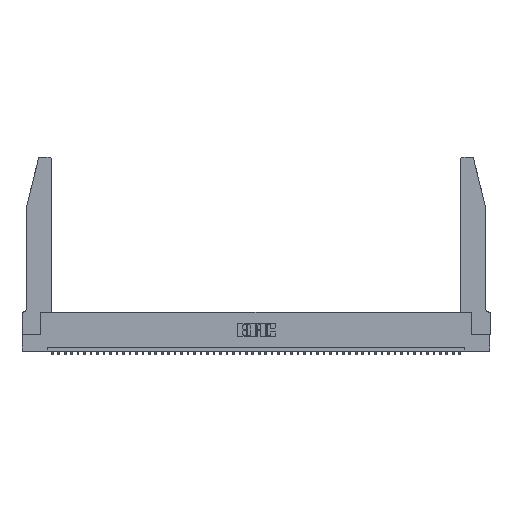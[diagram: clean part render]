
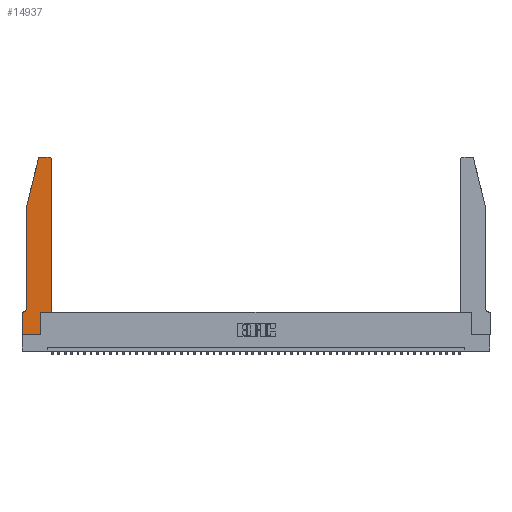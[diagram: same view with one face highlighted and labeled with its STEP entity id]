
A CAD part, top view. The second image highlights one B-rep face of the part: STEP entity #14937.
In plain terms, the highlighted planar face has unit normal (0, 0, 1).
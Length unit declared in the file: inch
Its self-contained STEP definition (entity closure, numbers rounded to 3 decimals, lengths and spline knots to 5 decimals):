
#186 = CARTESIAN_POINT ( 'NONE',  ( 0.0755, 0.35, 0.37 ) ) ;
#230 = AXIS2_PLACEMENT_3D ( 'NONE', #18281, #14562, #41820 ) ;
#433 = DIRECTION ( 'NONE',  ( -0.239, -0.971, 0. ) ) ;
#727 = EDGE_CURVE ( 'NONE', #13771, #45544, #39080, .T. ) ;
#1251 = FACE_OUTER_BOUND ( 'NONE', #7457, .T. ) ;
#2124 = CARTESIAN_POINT ( 'NONE',  ( 0., 0.35, 0.37 ) ) ;
#2493 = EDGE_CURVE ( 'NONE', #27347, #13121, #4326, .T. ) ;
#2676 = VECTOR ( 'NONE', #43701, 39.37008 ) ;
#3773 = CARTESIAN_POINT ( 'NONE',  ( 0.0055, 0.35, 0.37 ) ) ;
#3998 = EDGE_CURVE ( 'NONE', #44544, #13251, #23470, .T. ) ;
#4326 = LINE ( 'NONE', #32568, #39318 ) ;
#4371 = EDGE_CURVE ( 'NONE', #15235, #44544, #29997, .T. ) ;
#4794 = DIRECTION ( 'NONE',  ( 1., 0., 0. ) ) ;
#4804 = ORIENTED_EDGE ( 'NONE', *, *, #6406, .T. ) ;
#5043 = CARTESIAN_POINT ( 'NONE',  ( 0.0755, 2., 0.37 ) ) ;
#6080 = EDGE_CURVE ( 'NONE', #13251, #15840, #48644, .T. ) ;
#6301 = ORIENTED_EDGE ( 'NONE', *, *, #37651, .T. ) ;
#6406 = EDGE_CURVE ( 'NONE', #28997, #15235, #20868, .T. ) ;
#7157 = VECTOR ( 'NONE', #39104, 39.37008 ) ;
#7457 = EDGE_LOOP ( 'NONE', ( #36026, #28416, #6301, #4804, #25164, #46960, #48026, #23947, #49826, #29886, #9608, #45561 ) ) ;
#7654 = CARTESIAN_POINT ( 'NONE',  ( 0., 0., 0.37 ) ) ;
#8870 = CARTESIAN_POINT ( 'NONE',  ( 0.0055, 0.42, 0.37 ) ) ;
#9608 = ORIENTED_EDGE ( 'NONE', *, *, #43253, .T. ) ;
#10741 = EDGE_CURVE ( 'NONE', #34025, #13771, #33424, .T. ) ;
#11911 = CARTESIAN_POINT ( 'NONE',  ( 0., 0., 0.37 ) ) ;
#12797 = CARTESIAN_POINT ( 'NONE',  ( 0.4505, 0.35, 0.37 ) ) ;
#13121 = VERTEX_POINT ( 'NONE', #31941 ) ;
#13251 = VERTEX_POINT ( 'NONE', #31848 ) ;
#13439 = CARTESIAN_POINT ( 'NONE',  ( 0.25487, 2.72718, 0.37 ) ) ;
#13771 = VERTEX_POINT ( 'NONE', #49092 ) ;
#14562 = DIRECTION ( 'NONE',  ( 0., 0., 1. ) ) ;
#14937 = ADVANCED_FACE ( 'NONE', ( #1251 ), #21396, .T. ) ;
#15235 = VERTEX_POINT ( 'NONE', #36367 ) ;
#15744 = VECTOR ( 'NONE', #43638, 39.37008 ) ;
#15840 = VERTEX_POINT ( 'NONE', #7654 ) ;
#16369 = CARTESIAN_POINT ( 'NONE',  ( 0.4505, 0.35, 0.37 ) ) ;
#17500 = AXIS2_PLACEMENT_3D ( 'NONE', #18683, #18853, #41708 ) ;
#17698 = VERTEX_POINT ( 'NONE', #20449 ) ;
#18281 = CARTESIAN_POINT ( 'NONE',  ( 0.4205, 2.72, 0.37 ) ) ;
#18683 = CARTESIAN_POINT ( 'NONE',  ( 0.284, 2.72, 0.37 ) ) ;
#18853 = DIRECTION ( 'NONE',  ( 0., 0., 1. ) ) ;
#18910 = CIRCLE ( 'NONE', #230, 0.03 ) ;
#20019 = CARTESIAN_POINT ( 'NONE',  ( 0.2865, 0., 0.37 ) ) ;
#20449 = CARTESIAN_POINT ( 'NONE',  ( 0.4505, 2.72, 0.37 ) ) ;
#20547 = DIRECTION ( 'NONE',  ( 0., 0., -1. ) ) ;
#20868 = LINE ( 'NONE', #47381, #33464 ) ;
#21115 = DIRECTION ( 'NONE',  ( 0., -1., 0. ) ) ;
#21396 = PLANE ( 'NONE',  #47291 ) ;
#22083 = EDGE_CURVE ( 'NONE', #13121, #26865, #32556, .T. ) ;
#22107 = VECTOR ( 'NONE', #44521, 39.37008 ) ;
#23470 = LINE ( 'NONE', #186, #7157 ) ;
#23947 = ORIENTED_EDGE ( 'NONE', *, *, #37744, .T. ) ;
#24371 = DIRECTION ( 'NONE',  ( -1., 0., 0. ) ) ;
#24828 = CARTESIAN_POINT ( 'NONE',  ( 0.2865, 0.35, 0.37 ) ) ;
#25164 = ORIENTED_EDGE ( 'NONE', *, *, #4371, .T. ) ;
#25752 = LINE ( 'NONE', #42741, #40200 ) ;
#25969 = LINE ( 'NONE', #12797, #15744 ) ;
#26865 = VERTEX_POINT ( 'NONE', #13439 ) ;
#27347 = VERTEX_POINT ( 'NONE', #34919 ) ;
#28416 = ORIENTED_EDGE ( 'NONE', *, *, #22083, .T. ) ;
#28997 = VERTEX_POINT ( 'NONE', #5043 ) ;
#29886 = ORIENTED_EDGE ( 'NONE', *, *, #727, .T. ) ;
#29997 = CIRCLE ( 'NONE', #43450, 0.07 ) ;
#31848 = CARTESIAN_POINT ( 'NONE',  ( 0., 0.35, 0.37 ) ) ;
#31941 = CARTESIAN_POINT ( 'NONE',  ( 0.284, 2.75, 0.37 ) ) ;
#32556 = CIRCLE ( 'NONE', #17500, 0.03 ) ;
#32568 = CARTESIAN_POINT ( 'NONE',  ( 0.2605, 2.75, 0.37 ) ) ;
#33189 = CARTESIAN_POINT ( 'NONE',  ( 0., 0., 0.37 ) ) ;
#33424 = LINE ( 'NONE', #24828, #2676 ) ;
#33464 = VECTOR ( 'NONE', #21115, 39.37008 ) ;
#34025 = VERTEX_POINT ( 'NONE', #20019 ) ;
#34502 = EDGE_CURVE ( 'NONE', #17698, #27347, #18910, .T. ) ;
#34919 = CARTESIAN_POINT ( 'NONE',  ( 0.4205, 2.75, 0.37 ) ) ;
#35938 = CARTESIAN_POINT ( 'NONE',  ( 0.4505, 0.35, 0.37 ) ) ;
#36026 = ORIENTED_EDGE ( 'NONE', *, *, #2493, .T. ) ;
#36367 = CARTESIAN_POINT ( 'NONE',  ( 0.0755, 0.42, 0.37 ) ) ;
#37651 = EDGE_CURVE ( 'NONE', #26865, #28997, #25752, .T. ) ;
#37744 = EDGE_CURVE ( 'NONE', #15840, #34025, #45062, .T. ) ;
#39080 = LINE ( 'NONE', #35938, #46974 ) ;
#39104 = DIRECTION ( 'NONE',  ( -1., 0., 0. ) ) ;
#39318 = VECTOR ( 'NONE', #44226, 39.37008 ) ;
#40200 = VECTOR ( 'NONE', #433, 39.37008 ) ;
#41399 = VECTOR ( 'NONE', #45318, 39.37008 ) ;
#41708 = DIRECTION ( 'NONE',  ( 1., 0., 0. ) ) ;
#41820 = DIRECTION ( 'NONE',  ( 1., 0., 0. ) ) ;
#42741 = CARTESIAN_POINT ( 'NONE',  ( 0.0755, 2., 0.37 ) ) ;
#43253 = EDGE_CURVE ( 'NONE', #45544, #17698, #25969, .T. ) ;
#43450 = AXIS2_PLACEMENT_3D ( 'NONE', #8870, #20547, #24371 ) ;
#43638 = DIRECTION ( 'NONE',  ( 0., 1., 0. ) ) ;
#43701 = DIRECTION ( 'NONE',  ( 0., 1., 0. ) ) ;
#44226 = DIRECTION ( 'NONE',  ( -1., 0., 0. ) ) ;
#44521 = DIRECTION ( 'NONE',  ( 0., -1., 0. ) ) ;
#44544 = VERTEX_POINT ( 'NONE', #3773 ) ;
#45062 = LINE ( 'NONE', #11911, #41399 ) ;
#45318 = DIRECTION ( 'NONE',  ( 1., 0., 0. ) ) ;
#45544 = VERTEX_POINT ( 'NONE', #16369 ) ;
#45561 = ORIENTED_EDGE ( 'NONE', *, *, #34502, .T. ) ;
#46960 = ORIENTED_EDGE ( 'NONE', *, *, #3998, .T. ) ;
#46974 = VECTOR ( 'NONE', #4794, 39.37008 ) ;
#47291 = AXIS2_PLACEMENT_3D ( 'NONE', #2124, #49020, #48677 ) ;
#47381 = CARTESIAN_POINT ( 'NONE',  ( 0.0755, 2., 0.37 ) ) ;
#48026 = ORIENTED_EDGE ( 'NONE', *, *, #6080, .T. ) ;
#48644 = LINE ( 'NONE', #33189, #22107 ) ;
#48677 = DIRECTION ( 'NONE',  ( 1., 0., 0. ) ) ;
#49020 = DIRECTION ( 'NONE',  ( 0., 0., 1. ) ) ;
#49092 = CARTESIAN_POINT ( 'NONE',  ( 0.2865, 0.35, 0.37 ) ) ;
#49826 = ORIENTED_EDGE ( 'NONE', *, *, #10741, .T. ) ;
